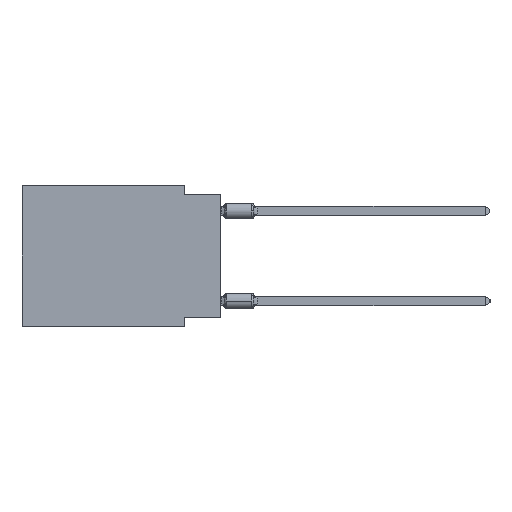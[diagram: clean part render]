
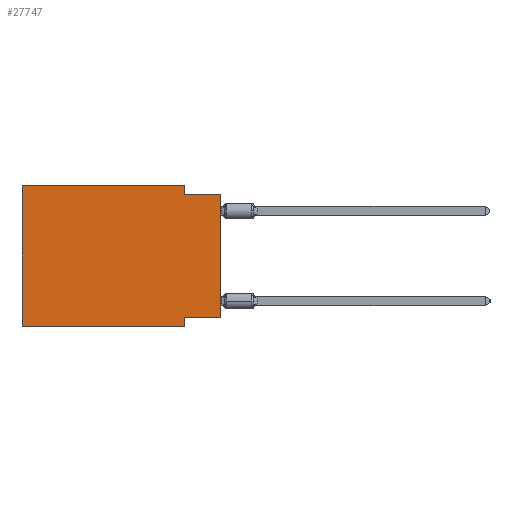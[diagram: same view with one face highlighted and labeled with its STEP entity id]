
A CAD part, left-side view. The second image highlights one B-rep face of the part: STEP entity #27747.
In plain terms, the highlighted planar face has unit normal (-1, 0, 0).
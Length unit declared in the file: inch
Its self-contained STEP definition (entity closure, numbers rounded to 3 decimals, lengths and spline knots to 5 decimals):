
#170 = CARTESIAN_POINT ( 'NONE',  ( 0., 0.55, 0. ) ) ;
#274 = EDGE_LOOP ( 'NONE', ( #14139, #26221, #12067, #22531, #39731, #17756, #11252, #11584 ) ) ;
#452 = CARTESIAN_POINT ( 'NONE',  ( 0., 0., -0.025 ) ) ;
#736 = DIRECTION ( 'NONE',  ( 0., 0., 1. ) ) ;
#774 = EDGE_CURVE ( 'NONE', #23916, #34915, #29101, .T. ) ;
#1252 = LINE ( 'NONE', #26756, #3079 ) ;
#1500 = CARTESIAN_POINT ( 'NONE',  ( 0., 0.1, -0.39 ) ) ;
#1728 = VECTOR ( 'NONE', #11011, 39.37008 ) ;
#2071 = DIRECTION ( 'NONE',  ( 0., 0., -1. ) ) ;
#2134 = DIRECTION ( 'NONE',  ( 0., 0., 1. ) ) ;
#2592 = EDGE_CURVE ( 'NONE', #39992, #10807, #1252, .T. ) ;
#2898 = EDGE_CURVE ( 'NONE', #22414, #39992, #28604, .T. ) ;
#3062 = DIRECTION ( 'NONE',  ( 0., -1., 0. ) ) ;
#3079 = VECTOR ( 'NONE', #13885, 39.37008 ) ;
#5183 = DIRECTION ( 'NONE',  ( 1., 0., 0. ) ) ;
#5647 = VERTEX_POINT ( 'NONE', #29842 ) ;
#6826 = VERTEX_POINT ( 'NONE', #452 ) ;
#6839 = AXIS2_PLACEMENT_3D ( 'NONE', #11383, #5183, #2071 ) ;
#7150 = CARTESIAN_POINT ( 'NONE',  ( 0., 0., 0. ) ) ;
#9062 = LINE ( 'NONE', #25029, #29271 ) ;
#10572 = VECTOR ( 'NONE', #39171, 39.37008 ) ;
#10807 = VERTEX_POINT ( 'NONE', #32850 ) ;
#11011 = DIRECTION ( 'NONE',  ( 0., 0., -1. ) ) ;
#11252 = ORIENTED_EDGE ( 'NONE', *, *, #774, .F. ) ;
#11383 = CARTESIAN_POINT ( 'NONE',  ( 0., 0.55, 0. ) ) ;
#11477 = CARTESIAN_POINT ( 'NONE',  ( 0., 0., -0.365 ) ) ;
#11584 = ORIENTED_EDGE ( 'NONE', *, *, #17263, .F. ) ;
#11701 = VECTOR ( 'NONE', #12797, 39.37008 ) ;
#12067 = ORIENTED_EDGE ( 'NONE', *, *, #2592, .F. ) ;
#12797 = DIRECTION ( 'NONE',  ( 0., -1., 0. ) ) ;
#13885 = DIRECTION ( 'NONE',  ( 0., 0., -1. ) ) ;
#13987 = DIRECTION ( 'NONE',  ( 0., 1., 0. ) ) ;
#14139 = ORIENTED_EDGE ( 'NONE', *, *, #19785, .T. ) ;
#14494 = PLANE ( 'NONE',  #6839 ) ;
#14591 = LINE ( 'NONE', #11477, #16281 ) ;
#14837 = VECTOR ( 'NONE', #2134, 39.37008 ) ;
#16281 = VECTOR ( 'NONE', #13987, 39.37008 ) ;
#16963 = LINE ( 'NONE', #35863, #10572 ) ;
#17263 = EDGE_CURVE ( 'NONE', #31261, #23916, #14591, .T. ) ;
#17756 = ORIENTED_EDGE ( 'NONE', *, *, #30690, .T. ) ;
#19785 = EDGE_CURVE ( 'NONE', #31261, #6826, #35581, .T. ) ;
#21046 = VECTOR ( 'NONE', #736, 39.37008 ) ;
#22414 = VERTEX_POINT ( 'NONE', #37533 ) ;
#22531 = ORIENTED_EDGE ( 'NONE', *, *, #2898, .F. ) ;
#23611 = EDGE_CURVE ( 'NONE', #10807, #6826, #16963, .T. ) ;
#23916 = VERTEX_POINT ( 'NONE', #30225 ) ;
#24531 = CARTESIAN_POINT ( 'NONE',  ( 0., 0.55, 0. ) ) ;
#25029 = CARTESIAN_POINT ( 'NONE',  ( 0., 0.55, -0.39 ) ) ;
#25709 = CARTESIAN_POINT ( 'NONE',  ( 0., 0.1, 0. ) ) ;
#26221 = ORIENTED_EDGE ( 'NONE', *, *, #23611, .F. ) ;
#26756 = CARTESIAN_POINT ( 'NONE',  ( 0., 0.1, 0. ) ) ;
#27747 = ADVANCED_FACE ( 'NONE', ( #30496 ), #14494, .F. ) ;
#28604 = LINE ( 'NONE', #170, #11701 ) ;
#29101 = LINE ( 'NONE', #1500, #1728 ) ;
#29271 = VECTOR ( 'NONE', #3062, 39.37008 ) ;
#29842 = CARTESIAN_POINT ( 'NONE',  ( 0., 0.55, -0.39 ) ) ;
#30225 = CARTESIAN_POINT ( 'NONE',  ( 0., 0.1, -0.365 ) ) ;
#30496 = FACE_OUTER_BOUND ( 'NONE', #274, .T. ) ;
#30690 = EDGE_CURVE ( 'NONE', #5647, #34915, #9062, .T. ) ;
#31261 = VERTEX_POINT ( 'NONE', #38479 ) ;
#32850 = CARTESIAN_POINT ( 'NONE',  ( 0., 0.1, -0.025 ) ) ;
#34277 = LINE ( 'NONE', #24531, #14837 ) ;
#34915 = VERTEX_POINT ( 'NONE', #40072 ) ;
#35581 = LINE ( 'NONE', #7150, #21046 ) ;
#35602 = EDGE_CURVE ( 'NONE', #5647, #22414, #34277, .T. ) ;
#35863 = CARTESIAN_POINT ( 'NONE',  ( 0., 0., -0.025 ) ) ;
#37533 = CARTESIAN_POINT ( 'NONE',  ( 0., 0.55, 0. ) ) ;
#38479 = CARTESIAN_POINT ( 'NONE',  ( 0., 0., -0.365 ) ) ;
#39171 = DIRECTION ( 'NONE',  ( 0., -1., 0. ) ) ;
#39731 = ORIENTED_EDGE ( 'NONE', *, *, #35602, .F. ) ;
#39992 = VERTEX_POINT ( 'NONE', #25709 ) ;
#40072 = CARTESIAN_POINT ( 'NONE',  ( 0., 0.1, -0.39 ) ) ;
